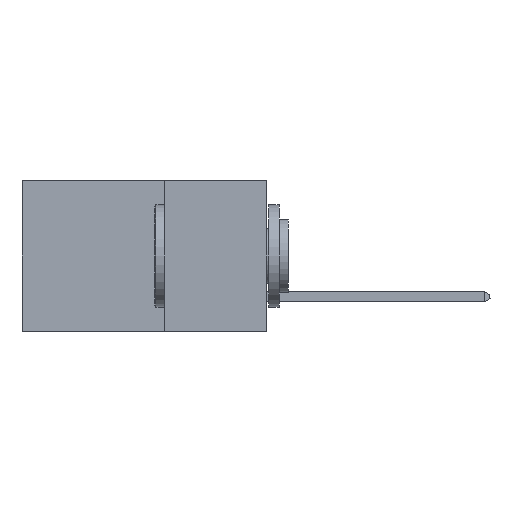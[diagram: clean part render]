
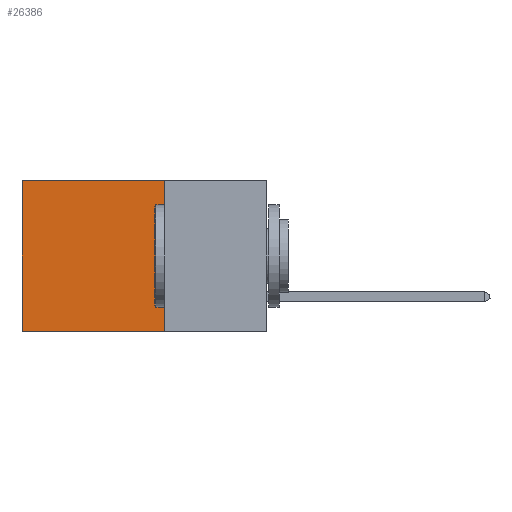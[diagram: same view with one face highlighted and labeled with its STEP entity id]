
A CAD part, left-side view. The second image highlights one B-rep face of the part: STEP entity #26386.
In plain terms, the highlighted planar face has unit normal (-1, 0, 0).
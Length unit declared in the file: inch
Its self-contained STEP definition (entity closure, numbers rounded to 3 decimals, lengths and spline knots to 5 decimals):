
#1997 = LINE ( 'NONE', #5686, #36001 ) ;
#2061 = FACE_OUTER_BOUND ( 'NONE', #35951, .T. ) ;
#2246 = CARTESIAN_POINT ( 'NONE',  ( 0.2875, 0.25, 0. ) ) ;
#3146 = VERTEX_POINT ( 'NONE', #35328 ) ;
#3332 = ORIENTED_EDGE ( 'NONE', *, *, #24338, .T. ) ;
#5243 = PLANE ( 'NONE',  #11227 ) ;
#5686 = CARTESIAN_POINT ( 'NONE',  ( 0.2875, 0.25, -0.37 ) ) ;
#6607 = LINE ( 'NONE', #29260, #9817 ) ;
#7699 = EDGE_CURVE ( 'NONE', #18895, #21472, #1997, .T. ) ;
#8200 = LINE ( 'NONE', #38355, #25471 ) ;
#9817 = VECTOR ( 'NONE', #29724, 39.37008 ) ;
#11227 = AXIS2_PLACEMENT_3D ( 'NONE', #2246, #25701, #29618 ) ;
#13307 = DIRECTION ( 'NONE',  ( 0., 0., -1. ) ) ;
#14955 = ORIENTED_EDGE ( 'NONE', *, *, #7699, .F. ) ;
#18807 = ORIENTED_EDGE ( 'NONE', *, *, #20870, .T. ) ;
#18895 = VERTEX_POINT ( 'NONE', #36485 ) ;
#19345 = DIRECTION ( 'NONE',  ( 0., 1., 0. ) ) ;
#20870 = EDGE_CURVE ( 'NONE', #21110, #3146, #6607, .T. ) ;
#21110 = VERTEX_POINT ( 'NONE', #35570 ) ;
#21472 = VERTEX_POINT ( 'NONE', #22529 ) ;
#22096 = ORIENTED_EDGE ( 'NONE', *, *, #28828, .F. ) ;
#22529 = CARTESIAN_POINT ( 'NONE',  ( 0.2875, 0.6, -0.37 ) ) ;
#23158 = VECTOR ( 'NONE', #13307, 39.37008 ) ;
#24338 = EDGE_CURVE ( 'NONE', #3146, #21472, #31796, .T. ) ;
#25471 = VECTOR ( 'NONE', #35302, 39.37008 ) ;
#25701 = DIRECTION ( 'NONE',  ( 1., 0., 0. ) ) ;
#26386 = ADVANCED_FACE ( 'NONE', ( #2061 ), #5243, .F. ) ;
#28828 = EDGE_CURVE ( 'NONE', #21110, #18895, #8200, .T. ) ;
#29260 = CARTESIAN_POINT ( 'NONE',  ( 0.2875, 0.25, 0. ) ) ;
#29618 = DIRECTION ( 'NONE',  ( 0., 0., -1. ) ) ;
#29724 = DIRECTION ( 'NONE',  ( 0., 1., 0. ) ) ;
#31796 = LINE ( 'NONE', #40582, #23158 ) ;
#35302 = DIRECTION ( 'NONE',  ( 0., 0., -1. ) ) ;
#35328 = CARTESIAN_POINT ( 'NONE',  ( 0.2875, 0.6, 0. ) ) ;
#35570 = CARTESIAN_POINT ( 'NONE',  ( 0.2875, 0.25, 0. ) ) ;
#35951 = EDGE_LOOP ( 'NONE', ( #3332, #14955, #22096, #18807 ) ) ;
#36001 = VECTOR ( 'NONE', #19345, 39.37008 ) ;
#36485 = CARTESIAN_POINT ( 'NONE',  ( 0.2875, 0.25, -0.37 ) ) ;
#38355 = CARTESIAN_POINT ( 'NONE',  ( 0.2875, 0.25, 0. ) ) ;
#40582 = CARTESIAN_POINT ( 'NONE',  ( 0.2875, 0.6, 0. ) ) ;
